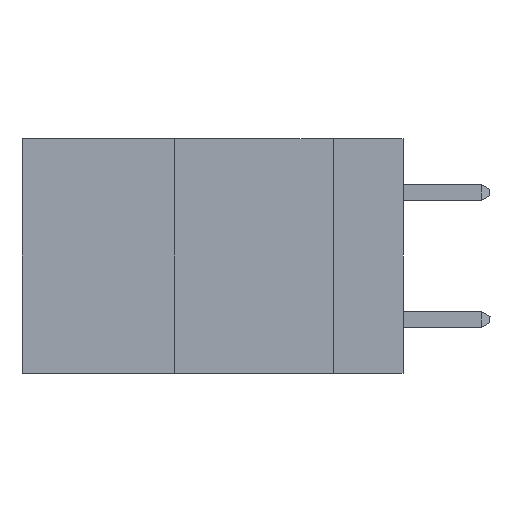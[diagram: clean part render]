
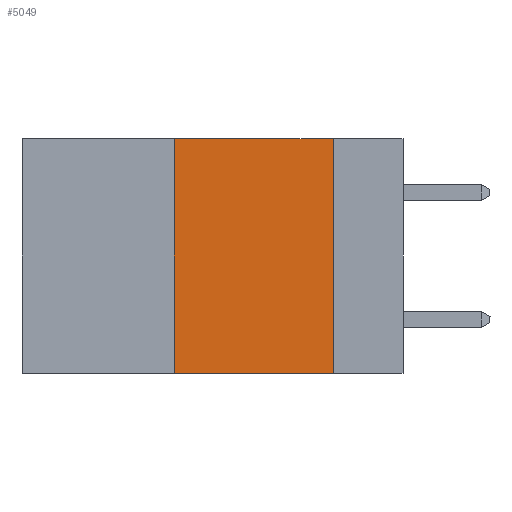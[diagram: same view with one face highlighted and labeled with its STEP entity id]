
A CAD part, left-side view. The second image highlights one B-rep face of the part: STEP entity #5049.
In plain terms, the highlighted planar face has unit normal (-1, 0, 0).
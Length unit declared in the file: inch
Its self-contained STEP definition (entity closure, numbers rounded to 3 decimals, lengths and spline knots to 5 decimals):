
#28 = CARTESIAN_POINT ( 'NONE',  ( 0., 0.36, 0. ) ) ;
#224 = ORIENTED_EDGE ( 'NONE', *, *, #1084, .F. ) ;
#409 = EDGE_CURVE ( 'NONE', #8355, #5788, #522, .T. ) ;
#522 = LINE ( 'NONE', #2007, #14652 ) ;
#613 = DIRECTION ( 'NONE',  ( 0., -1., 0. ) ) ;
#641 = VECTOR ( 'NONE', #2713, 39.37008 ) ;
#1084 = EDGE_CURVE ( 'NONE', #13596, #8355, #11060, .T. ) ;
#1351 = FACE_OUTER_BOUND ( 'NONE', #11200, .T. ) ;
#1632 = LINE ( 'NONE', #9721, #641 ) ;
#2007 = CARTESIAN_POINT ( 'NONE',  ( 0., 0.6, 0. ) ) ;
#2034 = VECTOR ( 'NONE', #12057, 39.37008 ) ;
#2713 = DIRECTION ( 'NONE',  ( 0., -1., 0. ) ) ;
#3320 = CARTESIAN_POINT ( 'NONE',  ( 0., 0.36, -0.37 ) ) ;
#4972 = CARTESIAN_POINT ( 'NONE',  ( 0., 0.36, 0. ) ) ;
#5049 = ADVANCED_FACE ( 'NONE', ( #1351 ), #11682, .F. ) ;
#5320 = CARTESIAN_POINT ( 'NONE',  ( 0., 0.11, 0. ) ) ;
#5788 = VERTEX_POINT ( 'NONE', #14832 ) ;
#5824 = LINE ( 'NONE', #5320, #5839 ) ;
#5839 = VECTOR ( 'NONE', #13836, 39.37008 ) ;
#7178 = ORIENTED_EDGE ( 'NONE', *, *, #12884, .T. ) ;
#8355 = VERTEX_POINT ( 'NONE', #28 ) ;
#8436 = VERTEX_POINT ( 'NONE', #13238 ) ;
#9435 = ORIENTED_EDGE ( 'NONE', *, *, #409, .F. ) ;
#9721 = CARTESIAN_POINT ( 'NONE',  ( 0., 0.6, -0.37 ) ) ;
#11060 = LINE ( 'NONE', #4972, #2034 ) ;
#11200 = EDGE_LOOP ( 'NONE', ( #12609, #9435, #224, #7178 ) ) ;
#11264 = AXIS2_PLACEMENT_3D ( 'NONE', #11911, #15327, #11767 ) ;
#11682 = PLANE ( 'NONE',  #11264 ) ;
#11767 = DIRECTION ( 'NONE',  ( 0., 0., -1. ) ) ;
#11911 = CARTESIAN_POINT ( 'NONE',  ( 0., 0.6, 0. ) ) ;
#12057 = DIRECTION ( 'NONE',  ( 0., 0., 1. ) ) ;
#12609 = ORIENTED_EDGE ( 'NONE', *, *, #14189, .F. ) ;
#12884 = EDGE_CURVE ( 'NONE', #13596, #8436, #1632, .T. ) ;
#13238 = CARTESIAN_POINT ( 'NONE',  ( 0., 0.11, -0.37 ) ) ;
#13596 = VERTEX_POINT ( 'NONE', #3320 ) ;
#13836 = DIRECTION ( 'NONE',  ( 0., 0., -1. ) ) ;
#14189 = EDGE_CURVE ( 'NONE', #5788, #8436, #5824, .T. ) ;
#14652 = VECTOR ( 'NONE', #613, 39.37008 ) ;
#14832 = CARTESIAN_POINT ( 'NONE',  ( 0., 0.11, 0. ) ) ;
#15327 = DIRECTION ( 'NONE',  ( 1., 0., 0. ) ) ;
